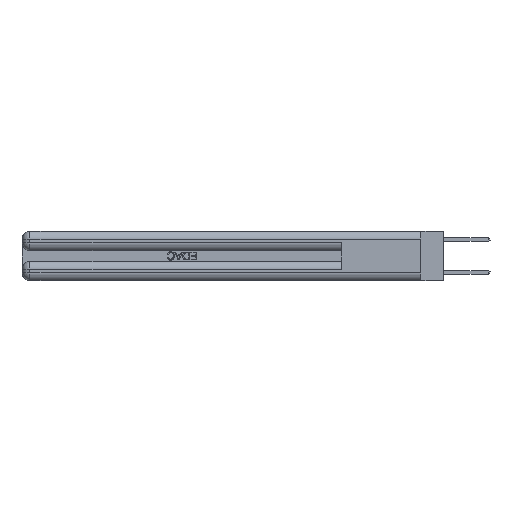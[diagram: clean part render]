
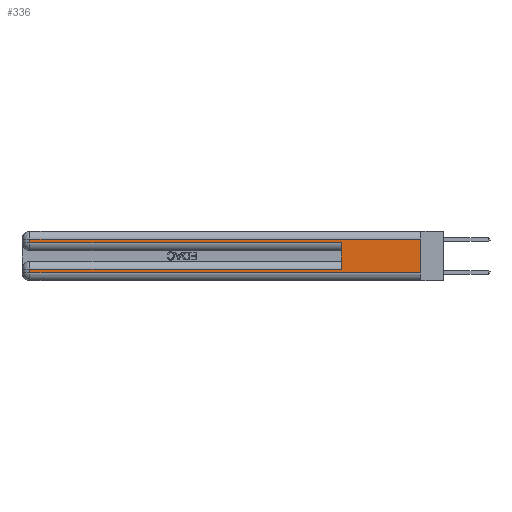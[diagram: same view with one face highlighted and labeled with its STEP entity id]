
A CAD part, left-side view. The second image highlights one B-rep face of the part: STEP entity #336.
In plain terms, the highlighted planar face has unit normal (-1, 0, 0).
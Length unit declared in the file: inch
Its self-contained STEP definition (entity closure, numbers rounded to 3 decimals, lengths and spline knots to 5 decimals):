
#236 = EDGE_CURVE ( 'NONE', #26017, #1907, #24456, .T. ) ;
#336 = ADVANCED_FACE ( 'NONE', ( #27634 ), #28374, .F. ) ;
#584 = CARTESIAN_POINT ( 'NONE',  ( 0., 0., 0.06 ) ) ;
#915 = DIRECTION ( 'NONE',  ( 0., 0., -1. ) ) ;
#1183 = ORIENTED_EDGE ( 'NONE', *, *, #3886, .T. ) ;
#1604 = DIRECTION ( 'NONE',  ( 0., 0., -1. ) ) ;
#1907 = VERTEX_POINT ( 'NONE', #15637 ) ;
#2736 = EDGE_CURVE ( 'NONE', #5593, #11624, #3330, .T. ) ;
#3330 = LINE ( 'NONE', #584, #9445 ) ;
#3886 = EDGE_CURVE ( 'NONE', #28106, #26017, #22678, .T. ) ;
#4089 = VERTEX_POINT ( 'NONE', #23854 ) ;
#4204 = VECTOR ( 'NONE', #23340, 39.37008 ) ;
#4349 = VECTOR ( 'NONE', #9491, 39.37008 ) ;
#4688 = DIRECTION ( 'NONE',  ( 0., 1., 0. ) ) ;
#4880 = CARTESIAN_POINT ( 'NONE',  ( 0., 2.94, 0.37 ) ) ;
#5108 = CARTESIAN_POINT ( 'NONE',  ( 0., 2.94, 0.37 ) ) ;
#5158 = DIRECTION ( 'NONE',  ( 0., -1., 0. ) ) ;
#5593 = VERTEX_POINT ( 'NONE', #13228 ) ;
#6142 = VECTOR ( 'NONE', #5158, 39.37008 ) ;
#6271 = EDGE_CURVE ( 'NONE', #21383, #1907, #16486, .T. ) ;
#6506 = CARTESIAN_POINT ( 'NONE',  ( 0., 0., 0.31 ) ) ;
#6802 = EDGE_CURVE ( 'NONE', #26456, #28106, #21784, .T. ) ;
#7300 = ORIENTED_EDGE ( 'NONE', *, *, #236, .T. ) ;
#8012 = ORIENTED_EDGE ( 'NONE', *, *, #17800, .T. ) ;
#8941 = CARTESIAN_POINT ( 'NONE',  ( 0., 0., 0.06 ) ) ;
#9445 = VECTOR ( 'NONE', #16717, 39.37008 ) ;
#9491 = DIRECTION ( 'NONE',  ( 0., 0., -1. ) ) ;
#10077 = CARTESIAN_POINT ( 'NONE',  ( 0., 0., 0.37 ) ) ;
#11059 = LINE ( 'NONE', #5108, #29276 ) ;
#11170 = CARTESIAN_POINT ( 'NONE',  ( 0., 0., 0.31 ) ) ;
#11211 = VECTOR ( 'NONE', #4688, 39.37008 ) ;
#11624 = VERTEX_POINT ( 'NONE', #8941 ) ;
#11939 = LINE ( 'NONE', #13839, #11211 ) ;
#13228 = CARTESIAN_POINT ( 'NONE',  ( 0., 2.94, 0.06 ) ) ;
#13839 = CARTESIAN_POINT ( 'NONE',  ( 0., 0., 0.085 ) ) ;
#14173 = ORIENTED_EDGE ( 'NONE', *, *, #28557, .T. ) ;
#14264 = DIRECTION ( 'NONE',  ( 0., 0., -1. ) ) ;
#14494 = EDGE_LOOP ( 'NONE', ( #24200, #18841, #1183, #7300, #19551, #8012, #14173, #20962 ) ) ;
#14726 = DIRECTION ( 'NONE',  ( 1., 0., 0. ) ) ;
#15637 = CARTESIAN_POINT ( 'NONE',  ( 0., 0.6, 0.285 ) ) ;
#16126 = CARTESIAN_POINT ( 'NONE',  ( 0., 2.94, 0.285 ) ) ;
#16486 = LINE ( 'NONE', #18554, #4204 ) ;
#16717 = DIRECTION ( 'NONE',  ( 0., -1., 0. ) ) ;
#17225 = CARTESIAN_POINT ( 'NONE',  ( 0., 2.94, 0.31 ) ) ;
#17800 = EDGE_CURVE ( 'NONE', #21383, #4089, #11939, .T. ) ;
#18093 = CARTESIAN_POINT ( 'NONE',  ( 0., 0.6, 0.085 ) ) ;
#18376 = LINE ( 'NONE', #19924, #29024 ) ;
#18554 = CARTESIAN_POINT ( 'NONE',  ( 0., 0.6, 0.145 ) ) ;
#18841 = ORIENTED_EDGE ( 'NONE', *, *, #6802, .T. ) ;
#19551 = ORIENTED_EDGE ( 'NONE', *, *, #6271, .F. ) ;
#19924 = CARTESIAN_POINT ( 'NONE',  ( 0., 0., 0.37 ) ) ;
#20962 = ORIENTED_EDGE ( 'NONE', *, *, #2736, .T. ) ;
#21065 = VECTOR ( 'NONE', #24904, 39.37008 ) ;
#21383 = VERTEX_POINT ( 'NONE', #18093 ) ;
#21784 = LINE ( 'NONE', #11170, #21065 ) ;
#22678 = LINE ( 'NONE', #4880, #4349 ) ;
#23340 = DIRECTION ( 'NONE',  ( 0., 0., 1. ) ) ;
#23854 = CARTESIAN_POINT ( 'NONE',  ( 0., 2.94, 0.085 ) ) ;
#24200 = ORIENTED_EDGE ( 'NONE', *, *, #25840, .F. ) ;
#24456 = LINE ( 'NONE', #25712, #6142 ) ;
#24904 = DIRECTION ( 'NONE',  ( 0., 1., 0. ) ) ;
#25144 = AXIS2_PLACEMENT_3D ( 'NONE', #10077, #14726, #915 ) ;
#25712 = CARTESIAN_POINT ( 'NONE',  ( 0., 0., 0.285 ) ) ;
#25840 = EDGE_CURVE ( 'NONE', #26456, #11624, #18376, .T. ) ;
#26017 = VERTEX_POINT ( 'NONE', #16126 ) ;
#26456 = VERTEX_POINT ( 'NONE', #6506 ) ;
#27634 = FACE_OUTER_BOUND ( 'NONE', #14494, .T. ) ;
#28106 = VERTEX_POINT ( 'NONE', #17225 ) ;
#28374 = PLANE ( 'NONE',  #25144 ) ;
#28557 = EDGE_CURVE ( 'NONE', #4089, #5593, #11059, .T. ) ;
#29024 = VECTOR ( 'NONE', #1604, 39.37008 ) ;
#29276 = VECTOR ( 'NONE', #14264, 39.37008 ) ;
